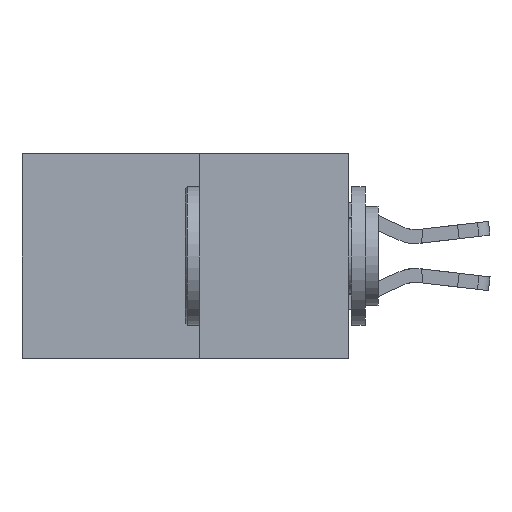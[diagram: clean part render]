
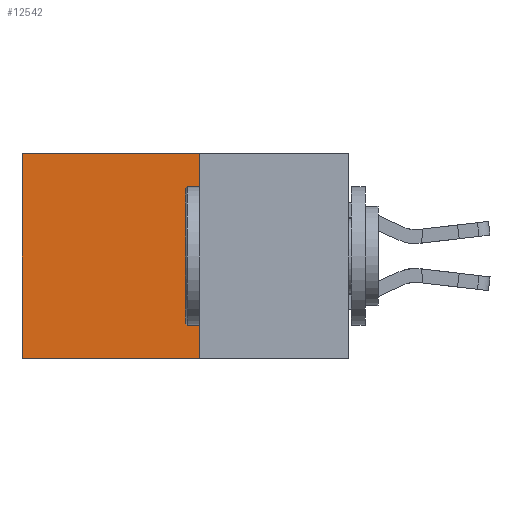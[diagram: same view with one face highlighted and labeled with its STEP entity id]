
A CAD part, left-side view. The second image highlights one B-rep face of the part: STEP entity #12542.
In plain terms, the highlighted planar face has unit normal (-1, 0, 0).
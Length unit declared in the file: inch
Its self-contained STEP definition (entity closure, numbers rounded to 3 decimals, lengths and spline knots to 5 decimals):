
#413 = CARTESIAN_POINT ( 'NONE',  ( 0.277, 0.27, -0.37 ) ) ;
#539 = VERTEX_POINT ( 'NONE', #413 ) ;
#953 = ORIENTED_EDGE ( 'NONE', *, *, #4877, .F. ) ;
#1973 = DIRECTION ( 'NONE',  ( 0., 1., 0. ) ) ;
#1980 = PLANE ( 'NONE',  #22342 ) ;
#2514 = LINE ( 'NONE', #3233, #7053 ) ;
#2668 = DIRECTION ( 'NONE',  ( 0., 0., -1. ) ) ;
#3233 = CARTESIAN_POINT ( 'NONE',  ( 0.277, 0.27, -0.37 ) ) ;
#4061 = CARTESIAN_POINT ( 'NONE',  ( 0.277, 0.59, -0.37 ) ) ;
#4877 = EDGE_CURVE ( 'NONE', #10046, #539, #2514, .T. ) ;
#4955 = EDGE_CURVE ( 'NONE', #5088, #22743, #14955, .T. ) ;
#5088 = VERTEX_POINT ( 'NONE', #24005 ) ;
#6361 = ORIENTED_EDGE ( 'NONE', *, *, #9732, .F. ) ;
#7053 = VECTOR ( 'NONE', #2668, 39.37008 ) ;
#7748 = CARTESIAN_POINT ( 'NONE',  ( 0.277, 0.27, -0.37 ) ) ;
#7794 = ORIENTED_EDGE ( 'NONE', *, *, #16029, .T. ) ;
#9732 = EDGE_CURVE ( 'NONE', #539, #22743, #10827, .T. ) ;
#9777 = DIRECTION ( 'NONE',  ( 1., 0., 0. ) ) ;
#9790 = VECTOR ( 'NONE', #21698, 39.37008 ) ;
#10046 = VERTEX_POINT ( 'NONE', #22335 ) ;
#10827 = LINE ( 'NONE', #7748, #14158 ) ;
#12542 = ADVANCED_FACE ( 'NONE', ( #22661 ), #1980, .F. ) ;
#14158 = VECTOR ( 'NONE', #23450, 39.37008 ) ;
#14955 = LINE ( 'NONE', #4061, #9790 ) ;
#16029 = EDGE_CURVE ( 'NONE', #10046, #5088, #23141, .T. ) ;
#17584 = ORIENTED_EDGE ( 'NONE', *, *, #4955, .T. ) ;
#17724 = CARTESIAN_POINT ( 'NONE',  ( 0.277, 0.59, -0.37 ) ) ;
#17888 = VECTOR ( 'NONE', #1973, 39.37008 ) ;
#19522 = CARTESIAN_POINT ( 'NONE',  ( 0.277, 0.27, -0.37 ) ) ;
#21698 = DIRECTION ( 'NONE',  ( 0., 0., -1. ) ) ;
#21982 = EDGE_LOOP ( 'NONE', ( #17584, #6361, #953, #7794 ) ) ;
#22335 = CARTESIAN_POINT ( 'NONE',  ( 0.277, 0.27, 0. ) ) ;
#22342 = AXIS2_PLACEMENT_3D ( 'NONE', #19522, #9777, #23523 ) ;
#22661 = FACE_OUTER_BOUND ( 'NONE', #21982, .T. ) ;
#22743 = VERTEX_POINT ( 'NONE', #17724 ) ;
#23141 = LINE ( 'NONE', #23521, #17888 ) ;
#23450 = DIRECTION ( 'NONE',  ( 0., 1., 0. ) ) ;
#23521 = CARTESIAN_POINT ( 'NONE',  ( 0.277, 0.27, 0. ) ) ;
#23523 = DIRECTION ( 'NONE',  ( 0., 0., -1. ) ) ;
#24005 = CARTESIAN_POINT ( 'NONE',  ( 0.277, 0.59, 0. ) ) ;
